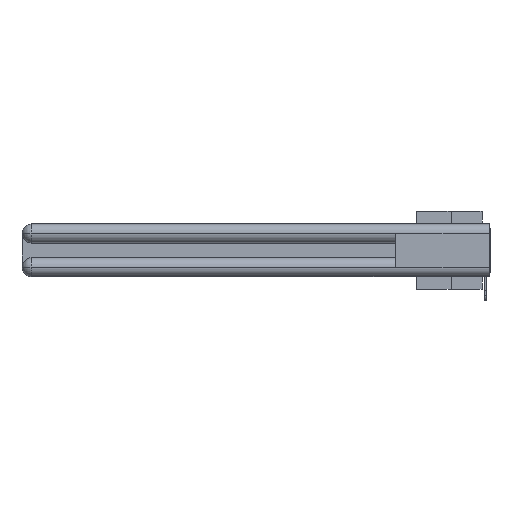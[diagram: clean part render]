
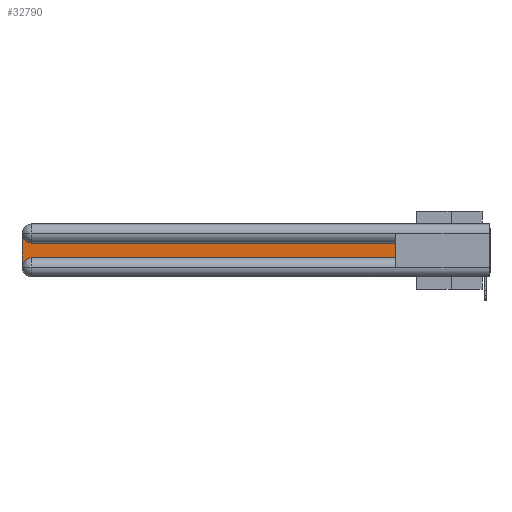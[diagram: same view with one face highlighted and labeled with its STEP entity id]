
A CAD part, left-side view. The second image highlights one B-rep face of the part: STEP entity #32790.
In plain terms, the highlighted planar face has unit normal (-1, 0, 0).
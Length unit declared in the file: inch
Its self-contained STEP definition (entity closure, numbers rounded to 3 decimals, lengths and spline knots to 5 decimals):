
#188 = DIRECTION ( 'NONE',  ( 0., 0., -1. ) ) ;
#857 = EDGE_LOOP ( 'NONE', ( #32046, #38550, #37092, #27188, #32558, #39846 ) ) ;
#1637 = DIRECTION ( 'NONE',  ( 0., 1., 0. ) ) ;
#3369 = DIRECTION ( 'NONE',  ( 1., 0., 0. ) ) ;
#4078 = VERTEX_POINT ( 'NONE', #21279 ) ;
#4652 = CARTESIAN_POINT ( 'NONE',  ( 0.075, 2.94, -0.0625 ) ) ;
#6104 = LINE ( 'NONE', #12218, #10655 ) ;
#6425 = CARTESIAN_POINT ( 'NONE',  ( 0.075, 2.94, -0.2775 ) ) ;
#7043 = DIRECTION ( 'NONE',  ( 0., 0., -1. ) ) ;
#7101 = AXIS2_PLACEMENT_3D ( 'NONE', #6425, #3369, #36826 ) ;
#7198 = VERTEX_POINT ( 'NONE', #20589 ) ;
#8544 = EDGE_CURVE ( 'NONE', #4078, #20781, #17528, .T. ) ;
#10427 = EDGE_CURVE ( 'NONE', #20781, #24333, #14344, .T. ) ;
#10655 = VECTOR ( 'NONE', #188, 39.37008 ) ;
#12218 = CARTESIAN_POINT ( 'NONE',  ( 0.075, 3., -0.2175 ) ) ;
#13556 = PLANE ( 'NONE',  #33328 ) ;
#14022 = DIRECTION ( 'NONE',  ( 0., 0., -1. ) ) ;
#14344 = CIRCLE ( 'NONE', #37162, 0.06 ) ;
#15344 = VERTEX_POINT ( 'NONE', #23038 ) ;
#15553 = VECTOR ( 'NONE', #36028, 39.37008 ) ;
#16431 = FACE_OUTER_BOUND ( 'NONE', #857, .T. ) ;
#17330 = CARTESIAN_POINT ( 'NONE',  ( 0.075, 0.6, -0.2175 ) ) ;
#17528 = LINE ( 'NONE', #29983, #18813 ) ;
#18017 = CARTESIAN_POINT ( 'NONE',  ( 0.075, 3., -0.0625 ) ) ;
#18813 = VECTOR ( 'NONE', #1637, 39.37008 ) ;
#18817 = CARTESIAN_POINT ( 'NONE',  ( 0.075, 2.94, -0.1225 ) ) ;
#19114 = EDGE_CURVE ( 'NONE', #7198, #15344, #37708, .T. ) ;
#19877 = DIRECTION ( 'NONE',  ( 1., 0., 0. ) ) ;
#20589 = CARTESIAN_POINT ( 'NONE',  ( 0.075, 3., -0.2775 ) ) ;
#20781 = VERTEX_POINT ( 'NONE', #18817 ) ;
#21279 = CARTESIAN_POINT ( 'NONE',  ( 0.075, 0.6, -0.1225 ) ) ;
#22967 = CARTESIAN_POINT ( 'NONE',  ( 0.075, 0.6, -0.2175 ) ) ;
#23038 = CARTESIAN_POINT ( 'NONE',  ( 0.075, 2.94, -0.2175 ) ) ;
#23673 = DIRECTION ( 'NONE',  ( 0., 0., 1. ) ) ;
#23774 = CARTESIAN_POINT ( 'NONE',  ( 0.075, 0.6, -0.2175 ) ) ;
#24333 = VERTEX_POINT ( 'NONE', #18017 ) ;
#25299 = EDGE_CURVE ( 'NONE', #24333, #7198, #6104, .T. ) ;
#25997 = CARTESIAN_POINT ( 'NONE',  ( 0.075, 3., -0.1225 ) ) ;
#27188 = ORIENTED_EDGE ( 'NONE', *, *, #19114, .T. ) ;
#27388 = VERTEX_POINT ( 'NONE', #22967 ) ;
#27765 = EDGE_CURVE ( 'NONE', #27388, #4078, #39179, .T. ) ;
#29983 = CARTESIAN_POINT ( 'NONE',  ( 0.075, 0.6, -0.1225 ) ) ;
#32046 = ORIENTED_EDGE ( 'NONE', *, *, #8544, .T. ) ;
#32558 = ORIENTED_EDGE ( 'NONE', *, *, #40350, .T. ) ;
#32790 = ADVANCED_FACE ( 'NONE', ( #16431 ), #13556, .F. ) ;
#32976 = DIRECTION ( 'NONE',  ( 1., 0., 0. ) ) ;
#33328 = AXIS2_PLACEMENT_3D ( 'NONE', #25997, #19877, #7043 ) ;
#34417 = VECTOR ( 'NONE', #23673, 39.37008 ) ;
#36028 = DIRECTION ( 'NONE',  ( 0., -1., 0. ) ) ;
#36826 = DIRECTION ( 'NONE',  ( 0., 0., -1. ) ) ;
#37092 = ORIENTED_EDGE ( 'NONE', *, *, #25299, .T. ) ;
#37162 = AXIS2_PLACEMENT_3D ( 'NONE', #4652, #32976, #14022 ) ;
#37708 = CIRCLE ( 'NONE', #7101, 0.06 ) ;
#38550 = ORIENTED_EDGE ( 'NONE', *, *, #10427, .T. ) ;
#39086 = LINE ( 'NONE', #23774, #15553 ) ;
#39179 = LINE ( 'NONE', #17330, #34417 ) ;
#39846 = ORIENTED_EDGE ( 'NONE', *, *, #27765, .T. ) ;
#40350 = EDGE_CURVE ( 'NONE', #15344, #27388, #39086, .T. ) ;
